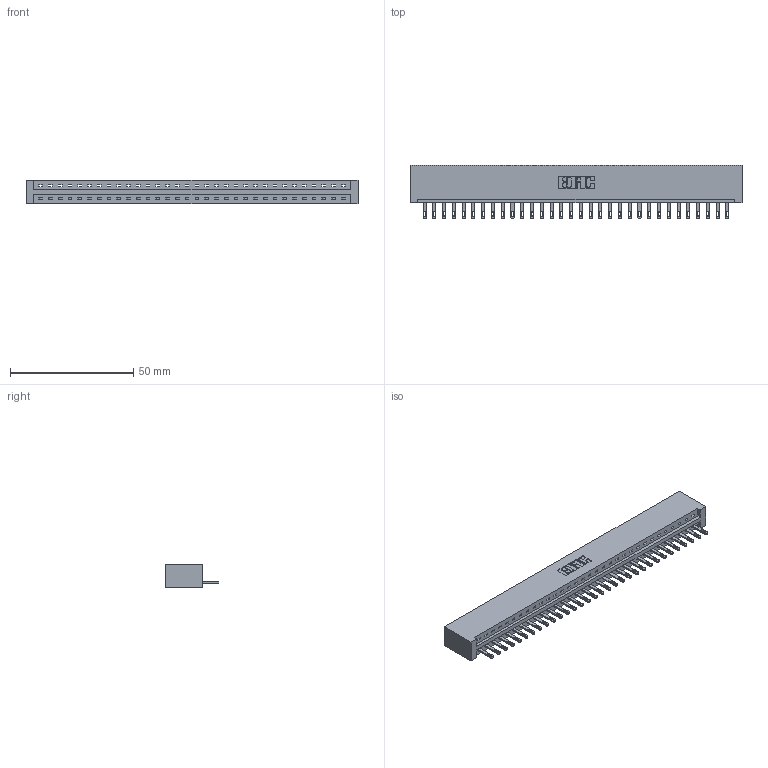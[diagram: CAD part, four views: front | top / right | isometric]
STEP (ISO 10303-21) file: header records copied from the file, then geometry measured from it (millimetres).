
FILE_DESCRIPTION (( 'STEP AP203' ), '1' );
FILE_NAME ('887-032-500-101.STEP', '2020-09-20T20:59:36', ( '' ), ( '' ), 'SwSTEP 2.0', 'SolidWorks 2020', '' );
FILE_SCHEMA (( 'CONFIG_CONTROL_DESIGN' ));
Length unit declared in the file: inch
Products named in the file (3): 837 Part_No Mounting Lugs; 887-032-500-101; 345-292-001_345-293-100
Assembly tree (33 placements, depth 2):
  887-032-500-101
    837 Part_No Mounting Lugs
    345-292-001_345-293-100  x32
Bounding box: 134.67 x 21.85 x 9.4 mm (x, y, z)
Volume: 14630.2 mm3; surface area: 15118.7 mm2
Topology: 33 solids, 33 shells, 1962 faces, 6047 edges, 4030 vertices
Faces by surface type: plane 1346, cylinder 616
Entity records: 24733 total; most frequent: CARTESIAN_POINT 4314, ORIENTED_EDGE 4282, DIRECTION 3645, EDGE_CURVE 2141, VECTOR 2017, LINE 2017, VERTEX_POINT 1426, AXIS2_PLACEMENT_3D 814
